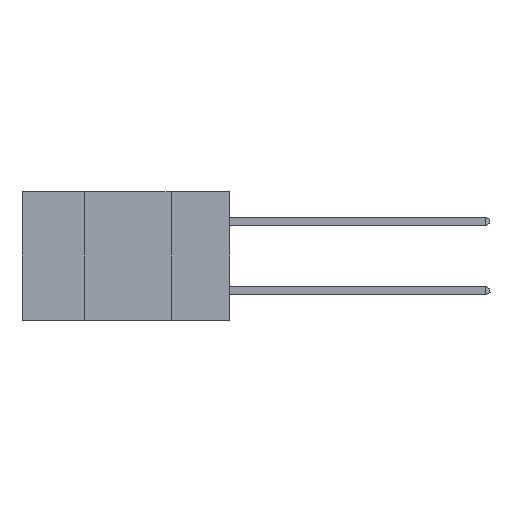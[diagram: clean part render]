
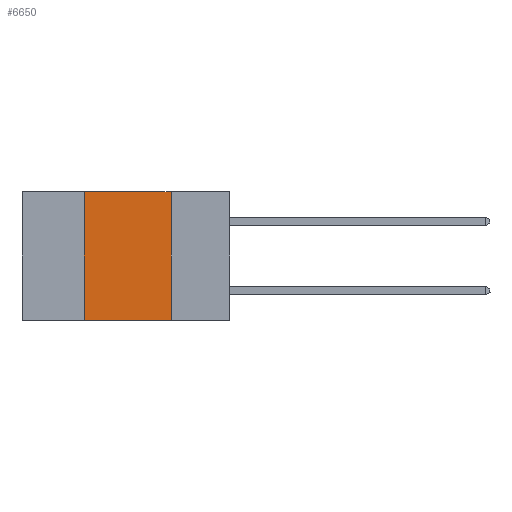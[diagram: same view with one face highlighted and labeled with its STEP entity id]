
A CAD part, left-side view. The second image highlights one B-rep face of the part: STEP entity #6650.
In plain terms, the highlighted planar face has unit normal (-1, 0, 0).
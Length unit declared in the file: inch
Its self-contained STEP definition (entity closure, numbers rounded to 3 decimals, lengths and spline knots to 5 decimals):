
#1002 = ORIENTED_EDGE ( 'NONE', *, *, #20432, .F. ) ;
#1062 = EDGE_CURVE ( 'NONE', #24572, #6682, #25012, .T. ) ;
#2611 = PLANE ( 'NONE',  #15708 ) ;
#3182 = ORIENTED_EDGE ( 'NONE', *, *, #26117, .F. ) ;
#4585 = ORIENTED_EDGE ( 'NONE', *, *, #1062, .T. ) ;
#4874 = LINE ( 'NONE', #28987, #21538 ) ;
#4892 = CARTESIAN_POINT ( 'NONE',  ( 0., 0.17, -0.37 ) ) ;
#5634 = VERTEX_POINT ( 'NONE', #21106 ) ;
#6650 = ADVANCED_FACE ( 'NONE', ( #15851 ), #2611, .F. ) ;
#6682 = VERTEX_POINT ( 'NONE', #4892 ) ;
#6860 = DIRECTION ( 'NONE',  ( 1., 0., 0. ) ) ;
#7557 = ORIENTED_EDGE ( 'NONE', *, *, #17231, .F. ) ;
#7702 = VERTEX_POINT ( 'NONE', #26209 ) ;
#7986 = VECTOR ( 'NONE', #25982, 39.37008 ) ;
#8186 = CARTESIAN_POINT ( 'NONE',  ( 0., 0.42, 0. ) ) ;
#8281 = DIRECTION ( 'NONE',  ( 0., 0., 1. ) ) ;
#9614 = DIRECTION ( 'NONE',  ( 0., -1., 0. ) ) ;
#9719 = CARTESIAN_POINT ( 'NONE',  ( 0., 0.6, 0. ) ) ;
#10662 = LINE ( 'NONE', #9719, #25231 ) ;
#15293 = CARTESIAN_POINT ( 'NONE',  ( 0., 0.42, -0.37 ) ) ;
#15303 = DIRECTION ( 'NONE',  ( 0., 0., -1. ) ) ;
#15708 = AXIS2_PLACEMENT_3D ( 'NONE', #20411, #6860, #18514 ) ;
#15851 = FACE_OUTER_BOUND ( 'NONE', #22646, .T. ) ;
#16639 = LINE ( 'NONE', #8186, #16984 ) ;
#16984 = VECTOR ( 'NONE', #8281, 39.37008 ) ;
#17231 = EDGE_CURVE ( 'NONE', #7702, #6682, #4874, .T. ) ;
#18514 = DIRECTION ( 'NONE',  ( 0., 0., -1. ) ) ;
#20411 = CARTESIAN_POINT ( 'NONE',  ( 0., 0.6, 0. ) ) ;
#20432 = EDGE_CURVE ( 'NONE', #24572, #5634, #16639, .T. ) ;
#21106 = CARTESIAN_POINT ( 'NONE',  ( 0., 0.42, 0. ) ) ;
#21538 = VECTOR ( 'NONE', #15303, 39.37008 ) ;
#22646 = EDGE_LOOP ( 'NONE', ( #7557, #3182, #1002, #4585 ) ) ;
#24572 = VERTEX_POINT ( 'NONE', #15293 ) ;
#25012 = LINE ( 'NONE', #26276, #7986 ) ;
#25231 = VECTOR ( 'NONE', #9614, 39.37008 ) ;
#25982 = DIRECTION ( 'NONE',  ( 0., -1., 0. ) ) ;
#26117 = EDGE_CURVE ( 'NONE', #5634, #7702, #10662, .T. ) ;
#26209 = CARTESIAN_POINT ( 'NONE',  ( 0., 0.17, 0. ) ) ;
#26276 = CARTESIAN_POINT ( 'NONE',  ( 0., 0.6, -0.37 ) ) ;
#28987 = CARTESIAN_POINT ( 'NONE',  ( 0., 0.17, 0. ) ) ;
